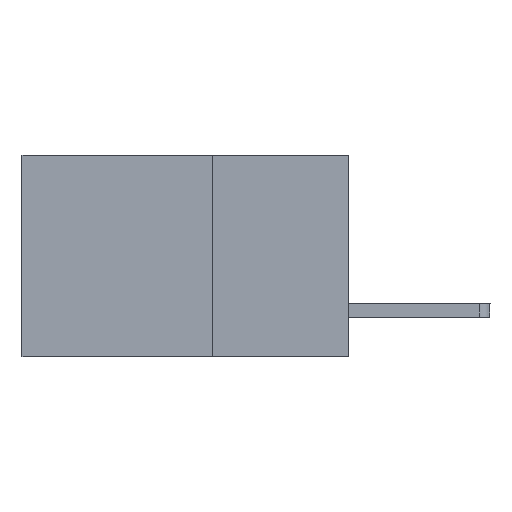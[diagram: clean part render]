
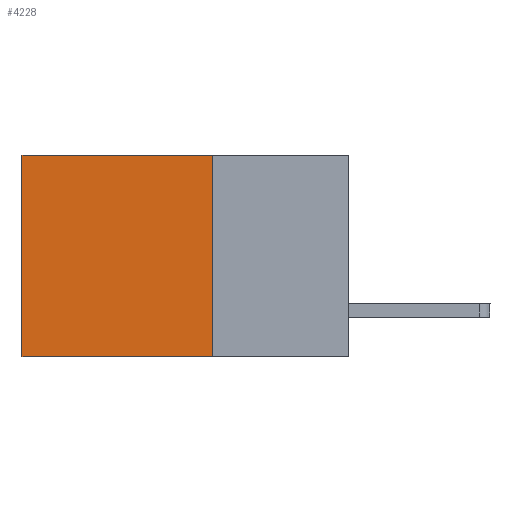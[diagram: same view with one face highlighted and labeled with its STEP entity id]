
A CAD part, left-side view. The second image highlights one B-rep face of the part: STEP entity #4228.
In plain terms, the highlighted planar face has unit normal (-1, 0, 0).
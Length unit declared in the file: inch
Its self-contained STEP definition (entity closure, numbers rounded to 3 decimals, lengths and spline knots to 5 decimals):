
#88 = DIRECTION ( 'NONE',  ( 0., 1., 0. ) ) ;
#223 = CARTESIAN_POINT ( 'NONE',  ( 0.2615, 0.25, 0. ) ) ;
#307 = DIRECTION ( 'NONE',  ( 0., 1., 0. ) ) ;
#402 = VERTEX_POINT ( 'NONE', #1112 ) ;
#832 = LINE ( 'NONE', #6251, #4985 ) ;
#1054 = EDGE_CURVE ( 'NONE', #6094, #5097, #4173, .T. ) ;
#1112 = CARTESIAN_POINT ( 'NONE',  ( 0.2615, 0.6, 0. ) ) ;
#1323 = DIRECTION ( 'NONE',  ( 0., 0., -1. ) ) ;
#1512 = ORIENTED_EDGE ( 'NONE', *, *, #4334, .T. ) ;
#1690 = EDGE_CURVE ( 'NONE', #8256, #6094, #5179, .T. ) ;
#2707 = DIRECTION ( 'NONE',  ( 1., 0., 0. ) ) ;
#2802 = ORIENTED_EDGE ( 'NONE', *, *, #1054, .F. ) ;
#2834 = CARTESIAN_POINT ( 'NONE',  ( 0.2615, 0.25, -0.37 ) ) ;
#3508 = AXIS2_PLACEMENT_3D ( 'NONE', #2834, #2707, #1323 ) ;
#4000 = VECTOR ( 'NONE', #8527, 39.37008 ) ;
#4173 = LINE ( 'NONE', #8290, #4572 ) ;
#4228 = ADVANCED_FACE ( 'NONE', ( #8036 ), #6119, .F. ) ;
#4334 = EDGE_CURVE ( 'NONE', #8256, #402, #832, .T. ) ;
#4572 = VECTOR ( 'NONE', #88, 39.37008 ) ;
#4685 = CARTESIAN_POINT ( 'NONE',  ( 0.2615, 0.6, -0.37 ) ) ;
#4694 = EDGE_CURVE ( 'NONE', #402, #5097, #4744, .T. ) ;
#4744 = LINE ( 'NONE', #7450, #7559 ) ;
#4985 = VECTOR ( 'NONE', #307, 39.37008 ) ;
#5046 = EDGE_LOOP ( 'NONE', ( #6138, #2802, #7996, #1512 ) ) ;
#5097 = VERTEX_POINT ( 'NONE', #4685 ) ;
#5125 = CARTESIAN_POINT ( 'NONE',  ( 0.2615, 0.25, -0.37 ) ) ;
#5179 = LINE ( 'NONE', #5125, #4000 ) ;
#6094 = VERTEX_POINT ( 'NONE', #8179 ) ;
#6109 = DIRECTION ( 'NONE',  ( 0., 0., -1. ) ) ;
#6119 = PLANE ( 'NONE',  #3508 ) ;
#6138 = ORIENTED_EDGE ( 'NONE', *, *, #4694, .T. ) ;
#6251 = CARTESIAN_POINT ( 'NONE',  ( 0.2615, 0.25, 0. ) ) ;
#7450 = CARTESIAN_POINT ( 'NONE',  ( 0.2615, 0.6, -0.37 ) ) ;
#7559 = VECTOR ( 'NONE', #6109, 39.37008 ) ;
#7996 = ORIENTED_EDGE ( 'NONE', *, *, #1690, .F. ) ;
#8036 = FACE_OUTER_BOUND ( 'NONE', #5046, .T. ) ;
#8179 = CARTESIAN_POINT ( 'NONE',  ( 0.2615, 0.25, -0.37 ) ) ;
#8256 = VERTEX_POINT ( 'NONE', #223 ) ;
#8290 = CARTESIAN_POINT ( 'NONE',  ( 0.2615, 0.25, -0.37 ) ) ;
#8527 = DIRECTION ( 'NONE',  ( 0., 0., -1. ) ) ;
